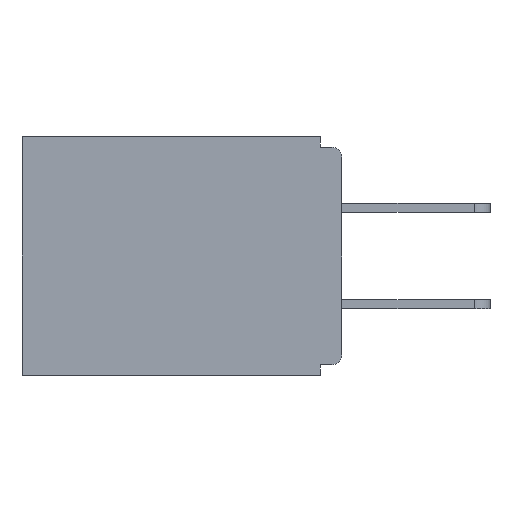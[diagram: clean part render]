
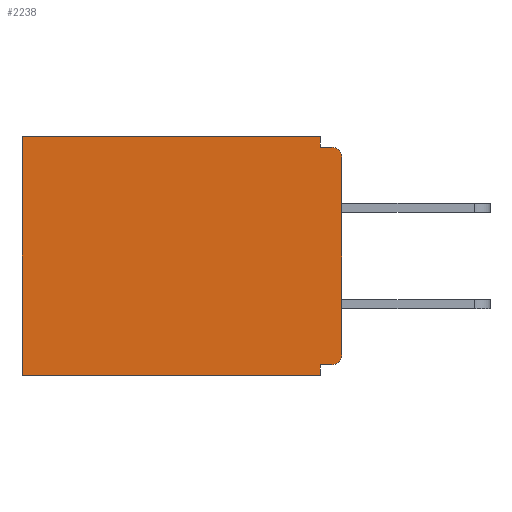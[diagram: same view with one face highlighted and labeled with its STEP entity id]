
A CAD part, left-side view. The second image highlights one B-rep face of the part: STEP entity #2238.
In plain terms, the highlighted planar face has unit normal (-1, 0, 0).
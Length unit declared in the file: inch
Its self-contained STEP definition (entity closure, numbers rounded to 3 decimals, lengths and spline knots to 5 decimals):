
#87 = DIRECTION ( 'NONE',  ( 0., 0., -1. ) ) ;
#692 = CARTESIAN_POINT ( 'NONE',  ( 0.298, 0.015, -0.015 ) ) ;
#701 = ORIENTED_EDGE ( 'NONE', *, *, #3773, .F. ) ;
#1502 = CARTESIAN_POINT ( 'NONE',  ( 0.298, 0., -0.343 ) ) ;
#2238 = ADVANCED_FACE ( 'NONE', ( #3930 ), #6652, .F. ) ;
#3208 = LINE ( 'NONE', #4448, #28334 ) ;
#3257 = EDGE_CURVE ( 'NONE', #22702, #25777, #27596, .T. ) ;
#3379 = LINE ( 'NONE', #24538, #13455 ) ;
#3499 = DIRECTION ( 'NONE',  ( 0., 1., 0. ) ) ;
#3642 = VERTEX_POINT ( 'NONE', #22278 ) ;
#3773 = EDGE_CURVE ( 'NONE', #12455, #11311, #5615, .T. ) ;
#3930 = FACE_OUTER_BOUND ( 'NONE', #24598, .T. ) ;
#4448 = CARTESIAN_POINT ( 'NONE',  ( 0.298, 0., -0.328 ) ) ;
#4559 = DIRECTION ( 'NONE',  ( -1., 0., 0. ) ) ;
#4595 = VECTOR ( 'NONE', #3499, 39.37008 ) ;
#4646 = CARTESIAN_POINT ( 'NONE',  ( 0.298, 0.015, -0.03 ) ) ;
#5615 = LINE ( 'NONE', #6824, #28639 ) ;
#5963 = CARTESIAN_POINT ( 'NONE',  ( 0.298, 0.031, -0.328 ) ) ;
#6231 = DIRECTION ( 'NONE',  ( 0., 1., 0. ) ) ;
#6309 = CARTESIAN_POINT ( 'NONE',  ( 0.298, 0.46, -0.343 ) ) ;
#6535 = DIRECTION ( 'NONE',  ( 0., 1., 0. ) ) ;
#6652 = PLANE ( 'NONE',  #12152 ) ;
#6824 = CARTESIAN_POINT ( 'NONE',  ( 0.298, 0.031, -0.343 ) ) ;
#6914 = DIRECTION ( 'NONE',  ( 0., 0., -1. ) ) ;
#7138 = DIRECTION ( 'NONE',  ( 0., 0., -1. ) ) ;
#7551 = CARTESIAN_POINT ( 'NONE',  ( 0.298, 0.015, -0.313 ) ) ;
#7675 = DIRECTION ( 'NONE',  ( 0., 0., -1. ) ) ;
#8103 = LINE ( 'NONE', #18761, #25757 ) ;
#8170 = LINE ( 'NONE', #9674, #29040 ) ;
#9213 = ORIENTED_EDGE ( 'NONE', *, *, #18156, .F. ) ;
#9239 = ORIENTED_EDGE ( 'NONE', *, *, #3257, .T. ) ;
#9281 = AXIS2_PLACEMENT_3D ( 'NONE', #4646, #4559, #7138 ) ;
#9674 = CARTESIAN_POINT ( 'NONE',  ( 0.298, 0., 0. ) ) ;
#9894 = ORIENTED_EDGE ( 'NONE', *, *, #14430, .T. ) ;
#10174 = DIRECTION ( 'NONE',  ( 0., 0., -1. ) ) ;
#10535 = EDGE_CURVE ( 'NONE', #15970, #26648, #3208, .T. ) ;
#10638 = CARTESIAN_POINT ( 'NONE',  ( 0.298, 0.031, 0. ) ) ;
#11245 = CARTESIAN_POINT ( 'NONE',  ( 0.298, 0.46, 0. ) ) ;
#11311 = VERTEX_POINT ( 'NONE', #13892 ) ;
#11623 = AXIS2_PLACEMENT_3D ( 'NONE', #7551, #23625, #12202 ) ;
#12121 = CARTESIAN_POINT ( 'NONE',  ( 0.298, 0.46, 0. ) ) ;
#12152 = AXIS2_PLACEMENT_3D ( 'NONE', #13813, #27560, #87 ) ;
#12202 = DIRECTION ( 'NONE',  ( 0., 0., -1. ) ) ;
#12455 = VERTEX_POINT ( 'NONE', #10638 ) ;
#12942 = VERTEX_POINT ( 'NONE', #692 ) ;
#13455 = VECTOR ( 'NONE', #17722, 39.37008 ) ;
#13813 = CARTESIAN_POINT ( 'NONE',  ( 0.298, 0., 0. ) ) ;
#13892 = CARTESIAN_POINT ( 'NONE',  ( 0.298, 0.031, -0.015 ) ) ;
#14430 = EDGE_CURVE ( 'NONE', #3642, #12942, #17667, .T. ) ;
#15369 = VECTOR ( 'NONE', #7675, 39.37008 ) ;
#15970 = VERTEX_POINT ( 'NONE', #20494 ) ;
#16543 = CARTESIAN_POINT ( 'NONE',  ( 0.298, 0.031, -0.343 ) ) ;
#16972 = EDGE_CURVE ( 'NONE', #3642, #24448, #8170, .T. ) ;
#17447 = LINE ( 'NONE', #1502, #18899 ) ;
#17667 = CIRCLE ( 'NONE', #9281, 0.015 ) ;
#17722 = DIRECTION ( 'NONE',  ( 0., 0., -1. ) ) ;
#17807 = ORIENTED_EDGE ( 'NONE', *, *, #16972, .F. ) ;
#18156 = EDGE_CURVE ( 'NONE', #24732, #25777, #17447, .T. ) ;
#18606 = LINE ( 'NONE', #19516, #4595 ) ;
#18666 = DIRECTION ( 'NONE',  ( 0., -1., 0. ) ) ;
#18761 = CARTESIAN_POINT ( 'NONE',  ( 0.298, 0., -0.015 ) ) ;
#18899 = VECTOR ( 'NONE', #6231, 39.37008 ) ;
#19516 = CARTESIAN_POINT ( 'NONE',  ( 0.298, 0., 0. ) ) ;
#19642 = ORIENTED_EDGE ( 'NONE', *, *, #23909, .T. ) ;
#20494 = CARTESIAN_POINT ( 'NONE',  ( 0.298, 0.015, -0.328 ) ) ;
#22151 = ORIENTED_EDGE ( 'NONE', *, *, #26721, .F. ) ;
#22278 = CARTESIAN_POINT ( 'NONE',  ( 0.298, 0., -0.03 ) ) ;
#22702 = VERTEX_POINT ( 'NONE', #11245 ) ;
#23194 = ORIENTED_EDGE ( 'NONE', *, *, #10535, .F. ) ;
#23625 = DIRECTION ( 'NONE',  ( -1., 0., 0. ) ) ;
#23909 = EDGE_CURVE ( 'NONE', #12455, #22702, #18606, .T. ) ;
#24448 = VERTEX_POINT ( 'NONE', #26612 ) ;
#24513 = CIRCLE ( 'NONE', #11623, 0.015 ) ;
#24538 = CARTESIAN_POINT ( 'NONE',  ( 0.298, 0.031, -0.343 ) ) ;
#24598 = EDGE_LOOP ( 'NONE', ( #9894, #26309, #701, #19642, #9239, #9213, #22151, #23194, #24854, #17807 ) ) ;
#24732 = VERTEX_POINT ( 'NONE', #16543 ) ;
#24854 = ORIENTED_EDGE ( 'NONE', *, *, #29181, .T. ) ;
#25757 = VECTOR ( 'NONE', #18666, 39.37008 ) ;
#25777 = VERTEX_POINT ( 'NONE', #6309 ) ;
#26309 = ORIENTED_EDGE ( 'NONE', *, *, #29703, .F. ) ;
#26612 = CARTESIAN_POINT ( 'NONE',  ( 0.298, 0., -0.313 ) ) ;
#26648 = VERTEX_POINT ( 'NONE', #5963 ) ;
#26721 = EDGE_CURVE ( 'NONE', #26648, #24732, #3379, .T. ) ;
#27560 = DIRECTION ( 'NONE',  ( 1., 0., 0. ) ) ;
#27596 = LINE ( 'NONE', #12121, #15369 ) ;
#28334 = VECTOR ( 'NONE', #6535, 39.37008 ) ;
#28639 = VECTOR ( 'NONE', #6914, 39.37008 ) ;
#29040 = VECTOR ( 'NONE', #10174, 39.37008 ) ;
#29181 = EDGE_CURVE ( 'NONE', #15970, #24448, #24513, .T. ) ;
#29703 = EDGE_CURVE ( 'NONE', #11311, #12942, #8103, .T. ) ;
